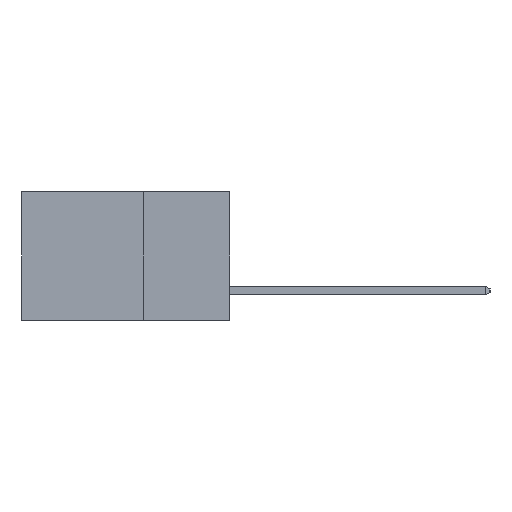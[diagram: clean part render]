
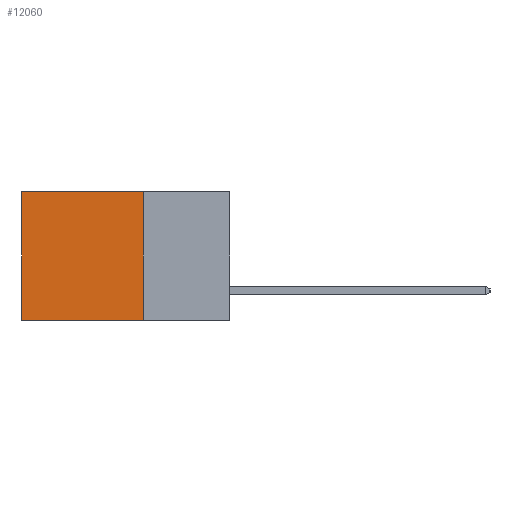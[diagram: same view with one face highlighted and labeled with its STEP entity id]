
A CAD part, left-side view. The second image highlights one B-rep face of the part: STEP entity #12060.
In plain terms, the highlighted planar face has unit normal (-1, 0, 0).
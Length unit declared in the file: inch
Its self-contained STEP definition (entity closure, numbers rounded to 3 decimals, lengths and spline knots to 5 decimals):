
#160 = EDGE_CURVE ( 'NONE', #25818, #26519, #1476, .T. ) ;
#856 = CARTESIAN_POINT ( 'NONE',  ( 0.298, 0.25, 0. ) ) ;
#985 = ORIENTED_EDGE ( 'NONE', *, *, #13208, .T. ) ;
#1476 = LINE ( 'NONE', #27339, #7505 ) ;
#2485 = CARTESIAN_POINT ( 'NONE',  ( 0.298, 0.25, 0. ) ) ;
#5436 = DIRECTION ( 'NONE',  ( 1., 0., 0. ) ) ;
#5860 = ORIENTED_EDGE ( 'NONE', *, *, #25760, .F. ) ;
#7505 = VECTOR ( 'NONE', #21639, 39.37008 ) ;
#7566 = VECTOR ( 'NONE', #13367, 39.37008 ) ;
#7641 = ORIENTED_EDGE ( 'NONE', *, *, #18247, .F. ) ;
#11153 = CARTESIAN_POINT ( 'NONE',  ( 0.298, 0.25, 0. ) ) ;
#12060 = ADVANCED_FACE ( 'NONE', ( #16811 ), #12075, .F. ) ;
#12075 = PLANE ( 'NONE',  #14603 ) ;
#12448 = EDGE_LOOP ( 'NONE', ( #21384, #7641, #5860, #985 ) ) ;
#13208 = EDGE_CURVE ( 'NONE', #22399, #25818, #25726, .T. ) ;
#13367 = DIRECTION ( 'NONE',  ( 0., 0., -1. ) ) ;
#13465 = CARTESIAN_POINT ( 'NONE',  ( 0.298, 0.6, 0. ) ) ;
#14603 = AXIS2_PLACEMENT_3D ( 'NONE', #856, #5436, #20905 ) ;
#14614 = VERTEX_POINT ( 'NONE', #18846 ) ;
#16811 = FACE_OUTER_BOUND ( 'NONE', #12448, .T. ) ;
#17007 = CARTESIAN_POINT ( 'NONE',  ( 0.298, 0.25, -0.37 ) ) ;
#18247 = EDGE_CURVE ( 'NONE', #14614, #26519, #26920, .T. ) ;
#18846 = CARTESIAN_POINT ( 'NONE',  ( 0.298, 0.25, -0.37 ) ) ;
#20144 = CARTESIAN_POINT ( 'NONE',  ( 0.298, 0.6, -0.37 ) ) ;
#20905 = DIRECTION ( 'NONE',  ( 0., 0., -1. ) ) ;
#21384 = ORIENTED_EDGE ( 'NONE', *, *, #160, .T. ) ;
#21616 = CARTESIAN_POINT ( 'NONE',  ( 0.298, 0.25, 0. ) ) ;
#21639 = DIRECTION ( 'NONE',  ( 0., 0., -1. ) ) ;
#21779 = VECTOR ( 'NONE', #28026, 39.37008 ) ;
#22399 = VERTEX_POINT ( 'NONE', #21616 ) ;
#25053 = VECTOR ( 'NONE', #26787, 39.37008 ) ;
#25165 = LINE ( 'NONE', #11153, #7566 ) ;
#25726 = LINE ( 'NONE', #2485, #25053 ) ;
#25760 = EDGE_CURVE ( 'NONE', #22399, #14614, #25165, .T. ) ;
#25818 = VERTEX_POINT ( 'NONE', #13465 ) ;
#26519 = VERTEX_POINT ( 'NONE', #20144 ) ;
#26787 = DIRECTION ( 'NONE',  ( 0., 1., 0. ) ) ;
#26920 = LINE ( 'NONE', #17007, #21779 ) ;
#27339 = CARTESIAN_POINT ( 'NONE',  ( 0.298, 0.6, 0. ) ) ;
#28026 = DIRECTION ( 'NONE',  ( 0., 1., 0. ) ) ;
